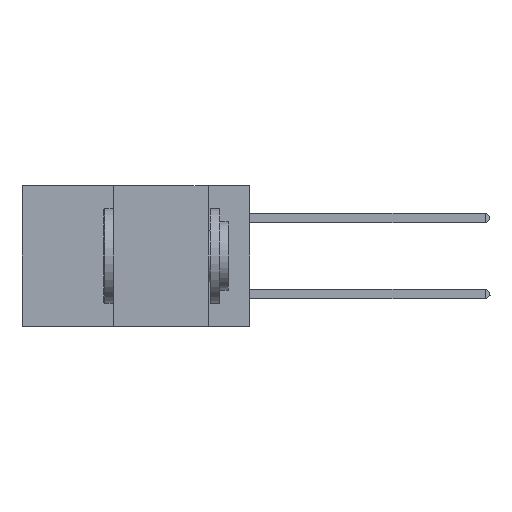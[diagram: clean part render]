
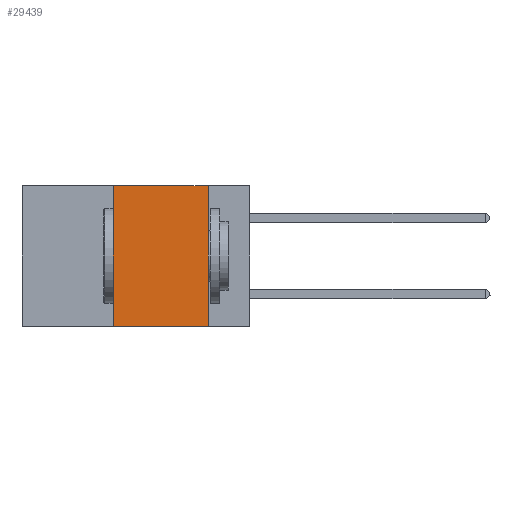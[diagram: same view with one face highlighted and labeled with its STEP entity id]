
A CAD part, left-side view. The second image highlights one B-rep face of the part: STEP entity #29439.
In plain terms, the highlighted planar face has unit normal (-1, 0, 0).
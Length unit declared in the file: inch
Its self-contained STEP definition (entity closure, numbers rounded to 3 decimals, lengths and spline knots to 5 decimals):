
#3782 = CARTESIAN_POINT ( 'NONE',  ( 0., 0.11, 0. ) ) ;
#3985 = ORIENTED_EDGE ( 'NONE', *, *, #19512, .F. ) ;
#5090 = EDGE_CURVE ( 'NONE', #19592, #10674, #33134, .T. ) ;
#5444 = EDGE_LOOP ( 'NONE', ( #31714, #5841, #3985, #26843 ) ) ;
#5841 = ORIENTED_EDGE ( 'NONE', *, *, #7262, .F. ) ;
#6503 = VERTEX_POINT ( 'NONE', #30616 ) ;
#7262 = EDGE_CURVE ( 'NONE', #6503, #19592, #10166, .T. ) ;
#7456 = DIRECTION ( 'NONE',  ( 0., -1., 0. ) ) ;
#8537 = DIRECTION ( 'NONE',  ( 0., 0., -1. ) ) ;
#10166 = LINE ( 'NONE', #22918, #32222 ) ;
#10610 = DIRECTION ( 'NONE',  ( 0., -1., 0. ) ) ;
#10674 = VERTEX_POINT ( 'NONE', #28313 ) ;
#11165 = CARTESIAN_POINT ( 'NONE',  ( 0., 0.36, 0. ) ) ;
#13077 = FACE_OUTER_BOUND ( 'NONE', #5444, .T. ) ;
#13228 = CARTESIAN_POINT ( 'NONE',  ( 0., 0.6, -0.37 ) ) ;
#13647 = DIRECTION ( 'NONE',  ( 1., 0., 0. ) ) ;
#16140 = DIRECTION ( 'NONE',  ( 0., 0., -1. ) ) ;
#17690 = LINE ( 'NONE', #13228, #22594 ) ;
#19512 = EDGE_CURVE ( 'NONE', #29251, #6503, #32333, .T. ) ;
#19592 = VERTEX_POINT ( 'NONE', #3782 ) ;
#21238 = PLANE ( 'NONE',  #33048 ) ;
#22594 = VECTOR ( 'NONE', #10610, 39.37008 ) ;
#22642 = CARTESIAN_POINT ( 'NONE',  ( 0., 0.36, -0.37 ) ) ;
#22918 = CARTESIAN_POINT ( 'NONE',  ( 0., 0.6, 0. ) ) ;
#23970 = CARTESIAN_POINT ( 'NONE',  ( 0., 0.6, 0. ) ) ;
#25801 = VECTOR ( 'NONE', #31906, 39.37008 ) ;
#26843 = ORIENTED_EDGE ( 'NONE', *, *, #33031, .T. ) ;
#28313 = CARTESIAN_POINT ( 'NONE',  ( 0., 0.11, -0.37 ) ) ;
#29251 = VERTEX_POINT ( 'NONE', #22642 ) ;
#29439 = ADVANCED_FACE ( 'NONE', ( #13077 ), #21238, .F. ) ;
#30616 = CARTESIAN_POINT ( 'NONE',  ( 0., 0.36, 0. ) ) ;
#31134 = CARTESIAN_POINT ( 'NONE',  ( 0., 0.11, 0. ) ) ;
#31491 = VECTOR ( 'NONE', #8537, 39.37008 ) ;
#31714 = ORIENTED_EDGE ( 'NONE', *, *, #5090, .F. ) ;
#31906 = DIRECTION ( 'NONE',  ( 0., 0., 1. ) ) ;
#32222 = VECTOR ( 'NONE', #7456, 39.37008 ) ;
#32333 = LINE ( 'NONE', #11165, #25801 ) ;
#33031 = EDGE_CURVE ( 'NONE', #29251, #10674, #17690, .T. ) ;
#33048 = AXIS2_PLACEMENT_3D ( 'NONE', #23970, #13647, #16140 ) ;
#33134 = LINE ( 'NONE', #31134, #31491 ) ;
